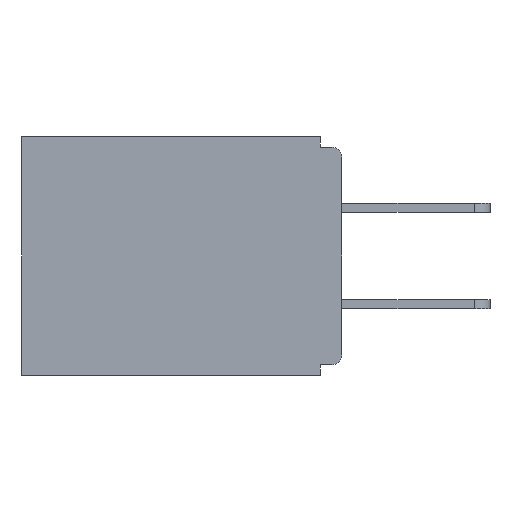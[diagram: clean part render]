
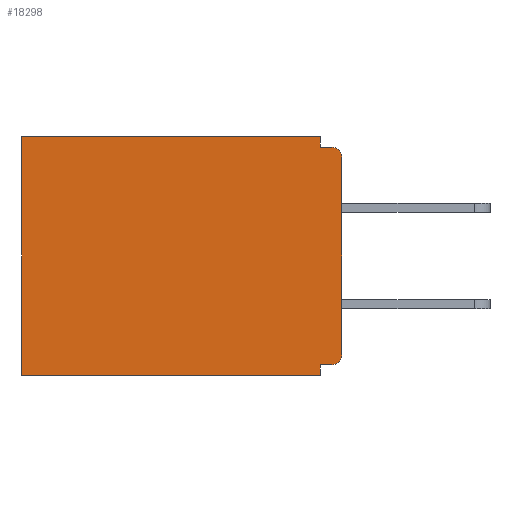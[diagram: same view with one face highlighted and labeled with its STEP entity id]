
A CAD part, left-side view. The second image highlights one B-rep face of the part: STEP entity #18298.
In plain terms, the highlighted planar face has unit normal (-1, 0, 0).
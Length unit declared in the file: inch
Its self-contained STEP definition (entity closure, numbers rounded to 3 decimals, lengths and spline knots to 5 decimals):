
#403 = ORIENTED_EDGE ( 'NONE', *, *, #11327, .T. ) ;
#449 = CARTESIAN_POINT ( 'NONE',  ( 0.298, 0., -0.343 ) ) ;
#538 = DIRECTION ( 'NONE',  ( 0., 0., -1. ) ) ;
#677 = ORIENTED_EDGE ( 'NONE', *, *, #5334, .T. ) ;
#1025 = EDGE_CURVE ( 'NONE', #15784, #17673, #12799, .T. ) ;
#1792 = VECTOR ( 'NONE', #9266, 39.37008 ) ;
#2120 = ORIENTED_EDGE ( 'NONE', *, *, #13547, .F. ) ;
#2545 = CIRCLE ( 'NONE', #12871, 0.015 ) ;
#2891 = CARTESIAN_POINT ( 'NONE',  ( 0.298, 0.46, 0. ) ) ;
#3107 = LINE ( 'NONE', #16761, #6949 ) ;
#3251 = VECTOR ( 'NONE', #10835, 39.37008 ) ;
#3689 = DIRECTION ( 'NONE',  ( 0., 1., 0. ) ) ;
#3696 = CARTESIAN_POINT ( 'NONE',  ( 0.298, 0., 0. ) ) ;
#3760 = CARTESIAN_POINT ( 'NONE',  ( 0.298, 0.46, -0.343 ) ) ;
#3951 = VECTOR ( 'NONE', #3689, 39.37008 ) ;
#4021 = VERTEX_POINT ( 'NONE', #10398 ) ;
#4196 = ORIENTED_EDGE ( 'NONE', *, *, #12856, .F. ) ;
#4456 = ORIENTED_EDGE ( 'NONE', *, *, #11492, .F. ) ;
#4529 = ORIENTED_EDGE ( 'NONE', *, *, #19512, .F. ) ;
#4683 = CARTESIAN_POINT ( 'NONE',  ( 0.298, 0., -0.328 ) ) ;
#5118 = AXIS2_PLACEMENT_3D ( 'NONE', #9616, #7962, #9755 ) ;
#5125 = VERTEX_POINT ( 'NONE', #16028 ) ;
#5334 = EDGE_CURVE ( 'NONE', #7303, #15784, #11081, .T. ) ;
#5904 = VERTEX_POINT ( 'NONE', #9516 ) ;
#5936 = CARTESIAN_POINT ( 'NONE',  ( 0.298, 0.031, -0.343 ) ) ;
#6433 = VERTEX_POINT ( 'NONE', #12160 ) ;
#6727 = PLANE ( 'NONE',  #9817 ) ;
#6949 = VECTOR ( 'NONE', #7119, 39.37008 ) ;
#7020 = VECTOR ( 'NONE', #8116, 39.37008 ) ;
#7119 = DIRECTION ( 'NONE',  ( 0., -1., 0. ) ) ;
#7197 = EDGE_LOOP ( 'NONE', ( #12046, #4529, #14919, #677, #16243, #4196, #4456, #15909, #403, #2120 ) ) ;
#7303 = VERTEX_POINT ( 'NONE', #18251 ) ;
#7962 = DIRECTION ( 'NONE',  ( -1., 0., 0. ) ) ;
#8116 = DIRECTION ( 'NONE',  ( 0., 1., 0. ) ) ;
#8235 = CARTESIAN_POINT ( 'NONE',  ( 0.298, 0., 0. ) ) ;
#8449 = CIRCLE ( 'NONE', #5118, 0.015 ) ;
#8546 = CARTESIAN_POINT ( 'NONE',  ( 0.298, 0.015, -0.313 ) ) ;
#8625 = DIRECTION ( 'NONE',  ( -1., 0., 0. ) ) ;
#8970 = VERTEX_POINT ( 'NONE', #20943 ) ;
#9266 = DIRECTION ( 'NONE',  ( 0., 0., -1. ) ) ;
#9304 = DIRECTION ( 'NONE',  ( 0., 0., -1. ) ) ;
#9516 = CARTESIAN_POINT ( 'NONE',  ( 0.298, 0.015, -0.328 ) ) ;
#9579 = LINE ( 'NONE', #4683, #10088 ) ;
#9616 = CARTESIAN_POINT ( 'NONE',  ( 0.298, 0.015, -0.03 ) ) ;
#9755 = DIRECTION ( 'NONE',  ( 0., 0., -1. ) ) ;
#9817 = AXIS2_PLACEMENT_3D ( 'NONE', #3696, #16923, #538 ) ;
#10088 = VECTOR ( 'NONE', #14308, 39.37008 ) ;
#10398 = CARTESIAN_POINT ( 'NONE',  ( 0.298, 0.031, -0.328 ) ) ;
#10835 = DIRECTION ( 'NONE',  ( 0., 0., -1. ) ) ;
#10862 = VERTEX_POINT ( 'NONE', #11148 ) ;
#11081 = LINE ( 'NONE', #11544, #7020 ) ;
#11148 = CARTESIAN_POINT ( 'NONE',  ( 0.298, 0., -0.313 ) ) ;
#11327 = EDGE_CURVE ( 'NONE', #5904, #10862, #2545, .T. ) ;
#11492 = EDGE_CURVE ( 'NONE', #4021, #12470, #15762, .T. ) ;
#11544 = CARTESIAN_POINT ( 'NONE',  ( 0.298, 0., 0. ) ) ;
#11822 = LINE ( 'NONE', #8235, #13603 ) ;
#12046 = ORIENTED_EDGE ( 'NONE', *, *, #14758, .T. ) ;
#12160 = CARTESIAN_POINT ( 'NONE',  ( 0.298, 0., -0.03 ) ) ;
#12275 = VECTOR ( 'NONE', #9304, 39.37008 ) ;
#12470 = VERTEX_POINT ( 'NONE', #17222 ) ;
#12546 = EDGE_CURVE ( 'NONE', #7303, #5125, #18285, .T. ) ;
#12799 = LINE ( 'NONE', #15631, #12275 ) ;
#12856 = EDGE_CURVE ( 'NONE', #12470, #17673, #20022, .T. ) ;
#12871 = AXIS2_PLACEMENT_3D ( 'NONE', #8546, #8625, #18161 ) ;
#13547 = EDGE_CURVE ( 'NONE', #6433, #10862, #11822, .T. ) ;
#13603 = VECTOR ( 'NONE', #19613, 39.37008 ) ;
#14308 = DIRECTION ( 'NONE',  ( 0., 1., 0. ) ) ;
#14758 = EDGE_CURVE ( 'NONE', #6433, #8970, #8449, .T. ) ;
#14919 = ORIENTED_EDGE ( 'NONE', *, *, #12546, .F. ) ;
#15631 = CARTESIAN_POINT ( 'NONE',  ( 0.298, 0.46, 0. ) ) ;
#15762 = LINE ( 'NONE', #20780, #1792 ) ;
#15784 = VERTEX_POINT ( 'NONE', #2891 ) ;
#15909 = ORIENTED_EDGE ( 'NONE', *, *, #18586, .F. ) ;
#16028 = CARTESIAN_POINT ( 'NONE',  ( 0.298, 0.031, -0.015 ) ) ;
#16200 = FACE_OUTER_BOUND ( 'NONE', #7197, .T. ) ;
#16243 = ORIENTED_EDGE ( 'NONE', *, *, #1025, .T. ) ;
#16761 = CARTESIAN_POINT ( 'NONE',  ( 0.298, 0., -0.015 ) ) ;
#16923 = DIRECTION ( 'NONE',  ( 1., 0., 0. ) ) ;
#17222 = CARTESIAN_POINT ( 'NONE',  ( 0.298, 0.031, -0.343 ) ) ;
#17673 = VERTEX_POINT ( 'NONE', #3760 ) ;
#18161 = DIRECTION ( 'NONE',  ( 0., 0., -1. ) ) ;
#18251 = CARTESIAN_POINT ( 'NONE',  ( 0.298, 0.031, 0. ) ) ;
#18285 = LINE ( 'NONE', #5936, #3251 ) ;
#18298 = ADVANCED_FACE ( 'NONE', ( #16200 ), #6727, .F. ) ;
#18586 = EDGE_CURVE ( 'NONE', #5904, #4021, #9579, .T. ) ;
#19512 = EDGE_CURVE ( 'NONE', #5125, #8970, #3107, .T. ) ;
#19613 = DIRECTION ( 'NONE',  ( 0., 0., -1. ) ) ;
#20022 = LINE ( 'NONE', #449, #3951 ) ;
#20780 = CARTESIAN_POINT ( 'NONE',  ( 0.298, 0.031, -0.343 ) ) ;
#20943 = CARTESIAN_POINT ( 'NONE',  ( 0.298, 0.015, -0.015 ) ) ;
